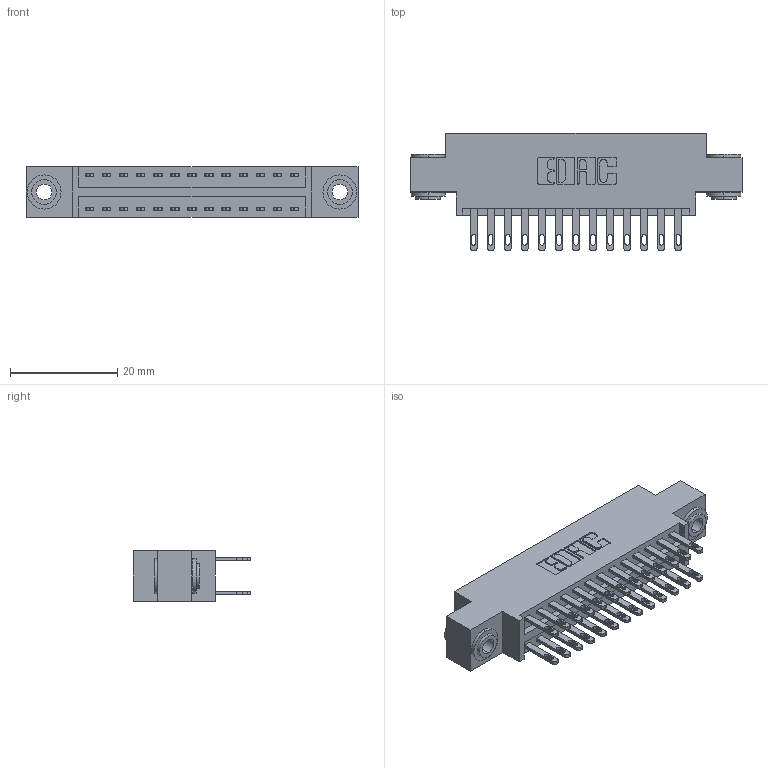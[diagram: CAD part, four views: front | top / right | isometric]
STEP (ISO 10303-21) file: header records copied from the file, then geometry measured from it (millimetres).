
FILE_DESCRIPTION (( 'STEP AP203' ), '1' );
FILE_NAME ('896-026-500-803.STEP', '2021-07-27T18:00:49', ( '' ), ( '' ), 'SwSTEP 2.0', 'SolidWorks 2020', '' );
FILE_SCHEMA (( 'CONFIG_CONTROL_DESIGN' ));
Length unit declared in the file: inch
Products named in the file (4): 896-026-500-803; 345-250-002_345-250-002-102; 345-292-001_345-293-100; 846 Part_0.170 Offset - 0.156 Dia-TH
Assembly tree (29 placements, depth 2):
  896-026-500-803
    846 Part_0.170 Offset - 0.156 Dia-TH
    345-292-001_345-293-100  x26
    345-250-002_345-250-002-102  x2
Bounding box: 61.85 x 21.84 x 9.4 mm (x, y, z)
Volume: 5750 mm3; surface area: 8113.9 mm2
Topology: 29 solids, 29 shells, 1412 faces, 4239 edges, 2822 vertices
Faces by surface type: plane 844, cylinder 560, cone 8
Entity records: 13100 total; most frequent: CARTESIAN_POINT 2175, ORIENTED_EDGE 2102, DIRECTION 2001, EDGE_CURVE 1051, VECTOR 839, LINE 839, VERTEX_POINT 698, AXIS2_PLACEMENT_3D 581
